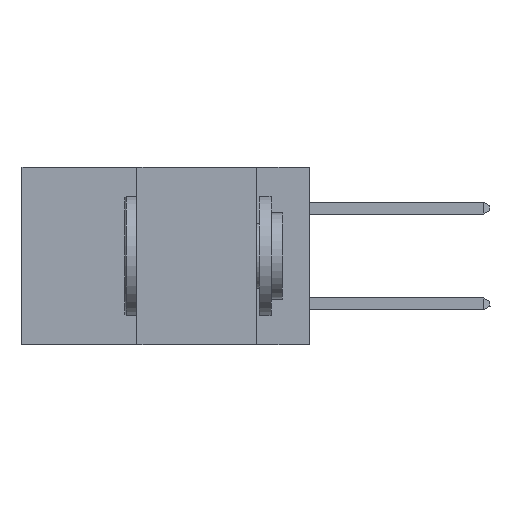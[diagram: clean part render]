
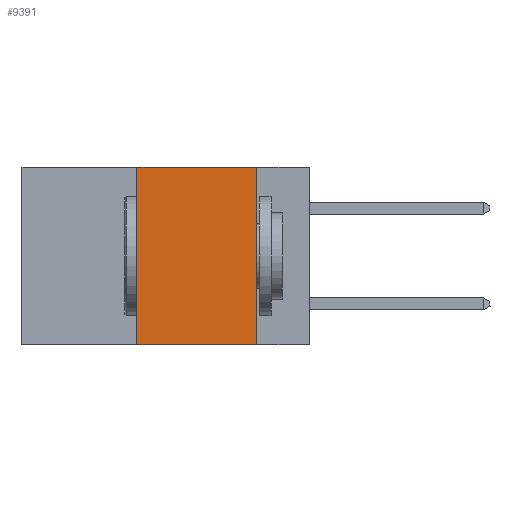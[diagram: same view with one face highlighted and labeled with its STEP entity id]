
A CAD part, left-side view. The second image highlights one B-rep face of the part: STEP entity #9391.
In plain terms, the highlighted planar face has unit normal (-1, 0, 0).
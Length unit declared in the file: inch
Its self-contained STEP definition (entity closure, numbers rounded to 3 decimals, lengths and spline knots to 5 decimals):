
#1966 = AXIS2_PLACEMENT_3D ( 'NONE', #42221, #25651, #19011 ) ;
#2147 = EDGE_CURVE ( 'NONE', #36761, #3832, #28939, .T. ) ;
#2784 = DIRECTION ( 'NONE',  ( 0., -1., 0. ) ) ;
#3832 = VERTEX_POINT ( 'NONE', #30204 ) ;
#4041 = ORIENTED_EDGE ( 'NONE', *, *, #39385, .F. ) ;
#5949 = PLANE ( 'NONE',  #1966 ) ;
#7174 = EDGE_LOOP ( 'NONE', ( #12556, #26122, #4041, #9331 ) ) ;
#9331 = ORIENTED_EDGE ( 'NONE', *, *, #18124, .T. ) ;
#9391 = ADVANCED_FACE ( 'NONE', ( #33433 ), #5949, .F. ) ;
#9571 = LINE ( 'NONE', #21658, #30153 ) ;
#11154 = VECTOR ( 'NONE', #25178, 39.37008 ) ;
#12556 = ORIENTED_EDGE ( 'NONE', *, *, #38880, .F. ) ;
#14352 = LINE ( 'NONE', #21122, #20149 ) ;
#15461 = CARTESIAN_POINT ( 'NONE',  ( 0., 0.6, -0.37 ) ) ;
#18124 = EDGE_CURVE ( 'NONE', #19157, #35668, #28028, .T. ) ;
#19011 = DIRECTION ( 'NONE',  ( 0., 0., -1. ) ) ;
#19157 = VERTEX_POINT ( 'NONE', #30279 ) ;
#20149 = VECTOR ( 'NONE', #41795, 39.37008 ) ;
#20495 = VECTOR ( 'NONE', #2784, 39.37008 ) ;
#21122 = CARTESIAN_POINT ( 'NONE',  ( 0., 0.11, 0. ) ) ;
#21658 = CARTESIAN_POINT ( 'NONE',  ( 0., 0.36, 0. ) ) ;
#22904 = CARTESIAN_POINT ( 'NONE',  ( 0., 0.6, 0. ) ) ;
#23399 = CARTESIAN_POINT ( 'NONE',  ( 0., 0.36, 0. ) ) ;
#25178 = DIRECTION ( 'NONE',  ( 0., -1., 0. ) ) ;
#25651 = DIRECTION ( 'NONE',  ( 1., 0., 0. ) ) ;
#26122 = ORIENTED_EDGE ( 'NONE', *, *, #2147, .F. ) ;
#27843 = CARTESIAN_POINT ( 'NONE',  ( 0., 0.11, -0.37 ) ) ;
#28028 = LINE ( 'NONE', #15461, #11154 ) ;
#28939 = LINE ( 'NONE', #22904, #20495 ) ;
#30153 = VECTOR ( 'NONE', #31983, 39.37008 ) ;
#30204 = CARTESIAN_POINT ( 'NONE',  ( 0., 0.11, 0. ) ) ;
#30279 = CARTESIAN_POINT ( 'NONE',  ( 0., 0.36, -0.37 ) ) ;
#31983 = DIRECTION ( 'NONE',  ( 0., 0., 1. ) ) ;
#33433 = FACE_OUTER_BOUND ( 'NONE', #7174, .T. ) ;
#35668 = VERTEX_POINT ( 'NONE', #27843 ) ;
#36761 = VERTEX_POINT ( 'NONE', #23399 ) ;
#38880 = EDGE_CURVE ( 'NONE', #3832, #35668, #14352, .T. ) ;
#39385 = EDGE_CURVE ( 'NONE', #19157, #36761, #9571, .T. ) ;
#41795 = DIRECTION ( 'NONE',  ( 0., 0., -1. ) ) ;
#42221 = CARTESIAN_POINT ( 'NONE',  ( 0., 0.6, 0. ) ) ;
